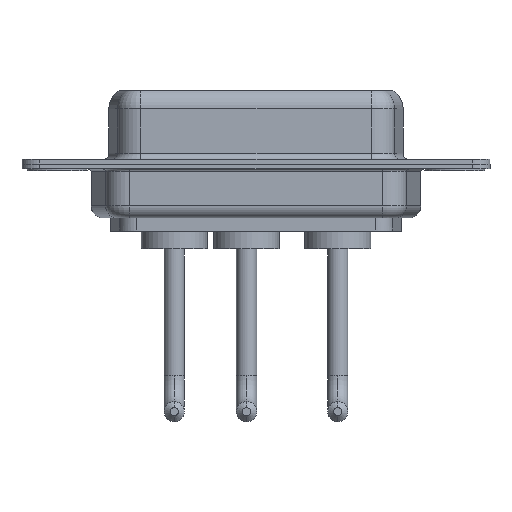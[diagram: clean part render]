
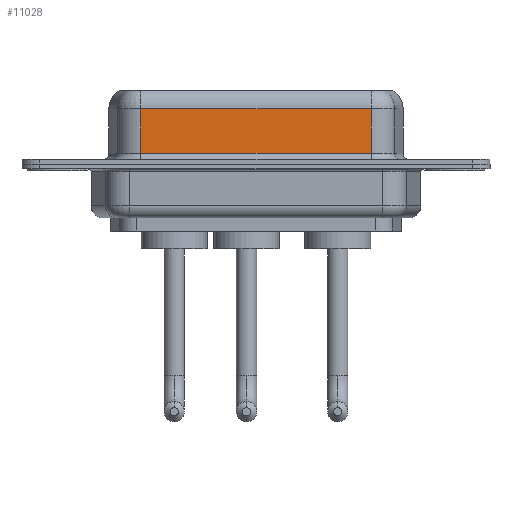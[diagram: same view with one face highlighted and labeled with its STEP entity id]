
A CAD part, front view. The second image highlights one B-rep face of the part: STEP entity #11028.
In plain terms, the highlighted planar face has unit normal (0, -1, 0).
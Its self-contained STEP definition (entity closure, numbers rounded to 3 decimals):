
#89 = ORIENTED_EDGE ( 'NONE', *, *, #5217, .F. ) ;
#221 = CARTESIAN_POINT ( 'NONE',  ( 26.287, -3.95, 6.4 ) ) ;
#456 = CARTESIAN_POINT ( 'NONE',  ( 26.287, -3.95, 4.65 ) ) ;
#811 = LINE ( 'NONE', #6380, #4161 ) ;
#1228 = EDGE_CURVE ( 'NONE', #11449, #9260, #1492, .T. ) ;
#1424 = DIRECTION ( 'NONE',  ( 1., 0., 0. ) ) ;
#1446 = VECTOR ( 'NONE', #9798, 1000. ) ;
#1492 = LINE ( 'NONE', #9801, #8519 ) ;
#2160 = DIRECTION ( 'NONE',  ( 0., 1., 0. ) ) ;
#2191 = CARTESIAN_POINT ( 'NONE',  ( 7.013, -3.95, 4.65 ) ) ;
#2250 = CARTESIAN_POINT ( 'NONE',  ( 7.013, -3.95, 6.4 ) ) ;
#2504 = AXIS2_PLACEMENT_3D ( 'NONE', #221, #2160, #9445 ) ;
#2704 = VERTEX_POINT ( 'NONE', #6435 ) ;
#3842 = PLANE ( 'NONE',  #2504 ) ;
#4161 = VECTOR ( 'NONE', #10081, 1000. ) ;
#4707 = EDGE_CURVE ( 'NONE', #2704, #8113, #7127, .T. ) ;
#5000 = ORIENTED_EDGE ( 'NONE', *, *, #5065, .T. ) ;
#5065 = EDGE_CURVE ( 'NONE', #8113, #11449, #8680, .T. ) ;
#5217 = EDGE_CURVE ( 'NONE', #2704, #9260, #811, .T. ) ;
#5943 = DIRECTION ( 'NONE',  ( 0., 0., -1. ) ) ;
#6380 = CARTESIAN_POINT ( 'NONE',  ( 26.287, -3.95, 6.4 ) ) ;
#6435 = CARTESIAN_POINT ( 'NONE',  ( 26.287, -3.95, 4.65 ) ) ;
#6795 = CARTESIAN_POINT ( 'NONE',  ( 7.013, -3.95, 0.9 ) ) ;
#7127 = LINE ( 'NONE', #456, #1446 ) ;
#7840 = CARTESIAN_POINT ( 'NONE',  ( 26.287, -3.95, 0.9 ) ) ;
#7847 = ORIENTED_EDGE ( 'NONE', *, *, #1228, .T. ) ;
#8113 = VERTEX_POINT ( 'NONE', #2191 ) ;
#8358 = FACE_OUTER_BOUND ( 'NONE', #10685, .T. ) ;
#8519 = VECTOR ( 'NONE', #1424, 1000. ) ;
#8680 = LINE ( 'NONE', #2250, #11925 ) ;
#9260 = VERTEX_POINT ( 'NONE', #7840 ) ;
#9445 = DIRECTION ( 'NONE',  ( 0., 0., 1. ) ) ;
#9798 = DIRECTION ( 'NONE',  ( -1., 0., 0. ) ) ;
#9801 = CARTESIAN_POINT ( 'NONE',  ( 26.287, -3.95, 0.9 ) ) ;
#10081 = DIRECTION ( 'NONE',  ( 0., 0., -1. ) ) ;
#10685 = EDGE_LOOP ( 'NONE', ( #89, #11654, #5000, #7847 ) ) ;
#11028 = ADVANCED_FACE ( 'NONE', ( #8358 ), #3842, .F. ) ;
#11449 = VERTEX_POINT ( 'NONE', #6795 ) ;
#11654 = ORIENTED_EDGE ( 'NONE', *, *, #4707, .T. ) ;
#11925 = VECTOR ( 'NONE', #5943, 1000. ) ;
